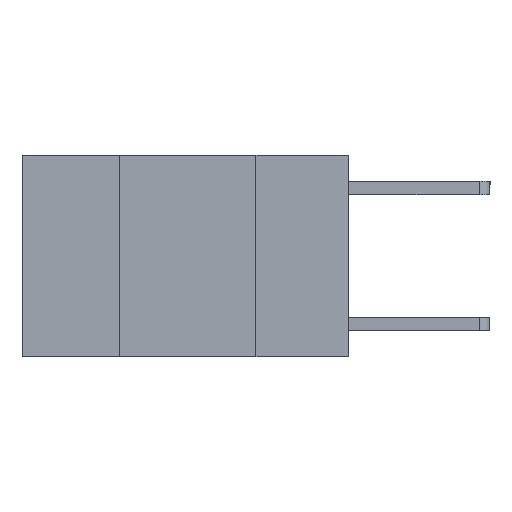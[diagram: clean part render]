
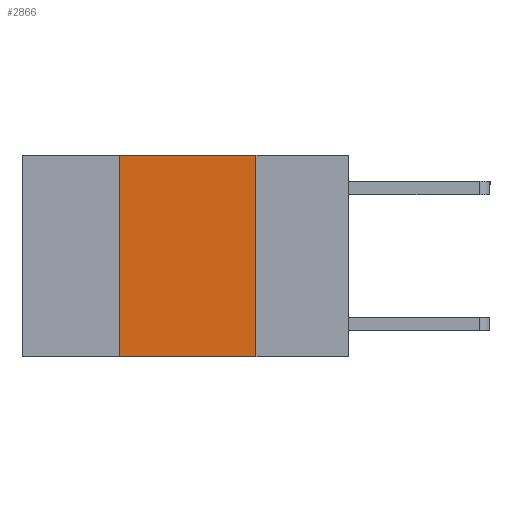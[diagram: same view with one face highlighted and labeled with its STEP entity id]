
A CAD part, left-side view. The second image highlights one B-rep face of the part: STEP entity #2866.
In plain terms, the highlighted planar face has unit normal (-1, 0, 0).
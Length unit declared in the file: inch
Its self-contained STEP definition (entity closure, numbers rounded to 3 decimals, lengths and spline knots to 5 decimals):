
#6 = ORIENTED_EDGE ( 'NONE', *, *, #10742, .F. ) ;
#230 = LINE ( 'NONE', #385, #6210 ) ;
#369 = DIRECTION ( 'NONE',  ( 0., -1., 0. ) ) ;
#385 = CARTESIAN_POINT ( 'NONE',  ( 0., 0.6, 0. ) ) ;
#402 = VERTEX_POINT ( 'NONE', #8130 ) ;
#1156 = DIRECTION ( 'NONE',  ( 1., 0., 0. ) ) ;
#1173 = VECTOR ( 'NONE', #369, 39.37008 ) ;
#1264 = FACE_OUTER_BOUND ( 'NONE', #6514, .T. ) ;
#1314 = VERTEX_POINT ( 'NONE', #3648 ) ;
#1610 = EDGE_CURVE ( 'NONE', #4704, #1314, #5477, .T. ) ;
#1637 = CARTESIAN_POINT ( 'NONE',  ( 0., 0.42, 0. ) ) ;
#1902 = ORIENTED_EDGE ( 'NONE', *, *, #7004, .F. ) ;
#2021 = CARTESIAN_POINT ( 'NONE',  ( 0., 0.6, -0.37 ) ) ;
#2866 = ADVANCED_FACE ( 'NONE', ( #1264 ), #9695, .F. ) ;
#3444 = VECTOR ( 'NONE', #10301, 39.37008 ) ;
#3648 = CARTESIAN_POINT ( 'NONE',  ( 0., 0.17, -0.37 ) ) ;
#4140 = CARTESIAN_POINT ( 'NONE',  ( 0., 0.42, -0.37 ) ) ;
#4250 = ORIENTED_EDGE ( 'NONE', *, *, #1610, .T. ) ;
#4377 = CARTESIAN_POINT ( 'NONE',  ( 0., 0.17, 0. ) ) ;
#4570 = LINE ( 'NONE', #4377, #3444 ) ;
#4651 = DIRECTION ( 'NONE',  ( 0., 0., -1. ) ) ;
#4704 = VERTEX_POINT ( 'NONE', #4140 ) ;
#5477 = LINE ( 'NONE', #2021, #1173 ) ;
#5730 = VECTOR ( 'NONE', #5754, 39.37008 ) ;
#5754 = DIRECTION ( 'NONE',  ( 0., 0., 1. ) ) ;
#6185 = CARTESIAN_POINT ( 'NONE',  ( 0., 0.42, 0. ) ) ;
#6210 = VECTOR ( 'NONE', #7769, 39.37008 ) ;
#6514 = EDGE_LOOP ( 'NONE', ( #7393, #1902, #6, #4250 ) ) ;
#6644 = LINE ( 'NONE', #1637, #5730 ) ;
#7004 = EDGE_CURVE ( 'NONE', #9105, #402, #230, .T. ) ;
#7393 = ORIENTED_EDGE ( 'NONE', *, *, #10428, .F. ) ;
#7603 = AXIS2_PLACEMENT_3D ( 'NONE', #9643, #1156, #4651 ) ;
#7769 = DIRECTION ( 'NONE',  ( 0., -1., 0. ) ) ;
#8130 = CARTESIAN_POINT ( 'NONE',  ( 0., 0.17, 0. ) ) ;
#9105 = VERTEX_POINT ( 'NONE', #6185 ) ;
#9643 = CARTESIAN_POINT ( 'NONE',  ( 0., 0.6, 0. ) ) ;
#9695 = PLANE ( 'NONE',  #7603 ) ;
#10301 = DIRECTION ( 'NONE',  ( 0., 0., -1. ) ) ;
#10428 = EDGE_CURVE ( 'NONE', #402, #1314, #4570, .T. ) ;
#10742 = EDGE_CURVE ( 'NONE', #4704, #9105, #6644, .T. ) ;
